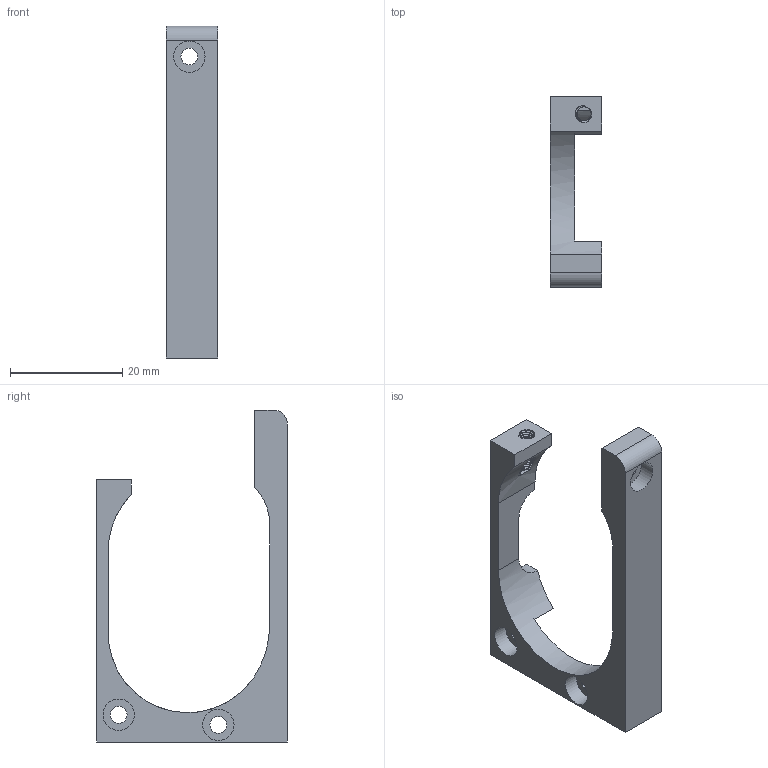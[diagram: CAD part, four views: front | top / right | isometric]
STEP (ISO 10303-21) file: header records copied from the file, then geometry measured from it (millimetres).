
FILE_DESCRIPTION(/* description */ (''),/* implementation_level */ '2;1');
FILE_NAME(/* name */ 'Right Trigger Guard.step',/* time_stamp */ '2024-01-16T15:55:36-05:00',/* author */ (''),/* organization */ (''),/* preprocessor_version */ 'ST-DEVELOPER v20',/* originating_system */ 'Autodesk Translation Framework v12.14.0.127',/* authorisation */ '');
FILE_SCHEMA (('AUTOMOTIVE_DESIGN { 1 0 10303 214 3 1 1 }'));
Length unit declared in the file: inch
Products named in the file (1): Right Trigger Guard
Bounding box: 9.22 x 34.06 x 59.26 mm (x, y, z)
Volume: 4154.6 mm3; surface area: 3568.4 mm2
Topology: 1 solids, 1 shells, 89 faces, 255 edges, 170 vertices
Faces by surface type: cylinder 51, plane 21, bspline 17
Full cylindrical faces by diameter (mm): 2.529 x6, 3 x3, 3.086 x4, 5.6 x3
Entity records: 4968 total; most frequent: CARTESIAN_POINT 2888, ORIENTED_EDGE 510, DIRECTION 284, EDGE_CURVE 255, VERTEX_POINT 170, B_SPLINE_CURVE_WITH_KNOTS 148, AXIS2_PLACEMENT_3D 104, EDGE_LOOP 101
